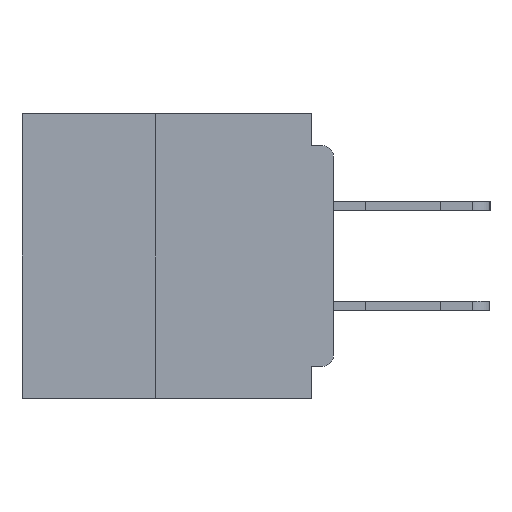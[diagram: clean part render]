
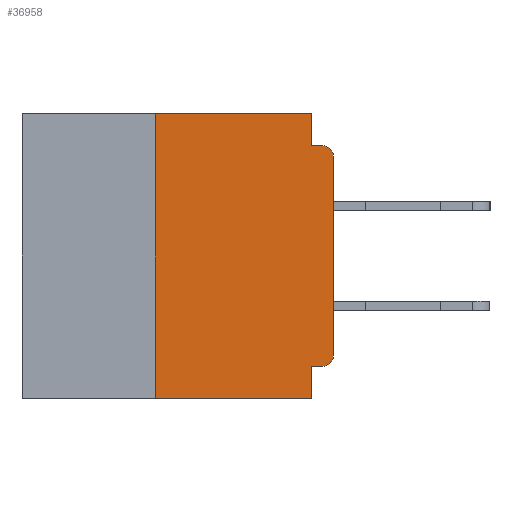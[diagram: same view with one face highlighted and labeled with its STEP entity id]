
A CAD part, left-side view. The second image highlights one B-rep face of the part: STEP entity #36958.
In plain terms, the highlighted planar face has unit normal (-1, 0, 0).
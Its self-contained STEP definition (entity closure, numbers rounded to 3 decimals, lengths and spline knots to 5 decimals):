
#415 = VECTOR ( 'NONE', #36513, 39.37008 ) ;
#615 = DIRECTION ( 'NONE',  ( 0., -1., 0. ) ) ;
#654 = CARTESIAN_POINT ( 'NONE',  ( 0., 0.015, -0.34 ) ) ;
#1583 = DIRECTION ( 'NONE',  ( -1., 0., 0. ) ) ;
#2540 = ORIENTED_EDGE ( 'NONE', *, *, #33725, .F. ) ;
#3178 = VECTOR ( 'NONE', #615, 39.37008 ) ;
#3676 = ORIENTED_EDGE ( 'NONE', *, *, #40113, .F. ) ;
#5214 = DIRECTION ( 'NONE',  ( 0., 0., 1. ) ) ;
#5276 = DIRECTION ( 'NONE',  ( 0., 0., -1. ) ) ;
#6387 = CARTESIAN_POINT ( 'NONE',  ( 0., 0.015, -0.355 ) ) ;
#6751 = CARTESIAN_POINT ( 'NONE',  ( 0., 0.031, 0. ) ) ;
#7031 = CARTESIAN_POINT ( 'NONE',  ( 0., 0.437, 0. ) ) ;
#7230 = DIRECTION ( 'NONE',  ( 0., 0., -1. ) ) ;
#7504 = LINE ( 'NONE', #15023, #29259 ) ;
#8085 = VERTEX_POINT ( 'NONE', #31874 ) ;
#8742 = ORIENTED_EDGE ( 'NONE', *, *, #43768, .T. ) ;
#8785 = EDGE_CURVE ( 'NONE', #26803, #26391, #31100, .T. ) ;
#8817 = CARTESIAN_POINT ( 'NONE',  ( 0., 0.25, 0. ) ) ;
#12615 = CARTESIAN_POINT ( 'NONE',  ( 0., 0.25, -0.4 ) ) ;
#13322 = LINE ( 'NONE', #33757, #37941 ) ;
#14015 = LINE ( 'NONE', #23815, #24891 ) ;
#15023 = CARTESIAN_POINT ( 'NONE',  ( 0., 0., -0.045 ) ) ;
#15478 = LINE ( 'NONE', #55989, #3178 ) ;
#17460 = LINE ( 'NONE', #35162, #52956 ) ;
#19173 = EDGE_CURVE ( 'NONE', #26803, #22892, #51169, .T. ) ;
#19683 = VERTEX_POINT ( 'NONE', #24675 ) ;
#20898 = CIRCLE ( 'NONE', #54994, 0.015 ) ;
#22050 = DIRECTION ( 'NONE',  ( 0., 0., -1. ) ) ;
#22139 = ORIENTED_EDGE ( 'NONE', *, *, #57718, .T. ) ;
#22577 = CARTESIAN_POINT ( 'NONE',  ( 0., 0.031, -0.355 ) ) ;
#22752 = CARTESIAN_POINT ( 'NONE',  ( 0., 0., 0. ) ) ;
#22892 = VERTEX_POINT ( 'NONE', #22577 ) ;
#23282 = VERTEX_POINT ( 'NONE', #6751 ) ;
#23600 = ORIENTED_EDGE ( 'NONE', *, *, #58479, .F. ) ;
#23815 = CARTESIAN_POINT ( 'NONE',  ( 0., 0.25, -0.4 ) ) ;
#24147 = ORIENTED_EDGE ( 'NONE', *, *, #53284, .F. ) ;
#24404 = EDGE_LOOP ( 'NONE', ( #22139, #8742, #3676, #28095, #24147, #23600, #30079, #2540, #34623, #55892 ) ) ;
#24675 = CARTESIAN_POINT ( 'NONE',  ( 0., 0.031, -0.045 ) ) ;
#24826 = CARTESIAN_POINT ( 'NONE',  ( 0., 0.031, -0.4 ) ) ;
#24891 = VECTOR ( 'NONE', #5214, 39.37008 ) ;
#25658 = PLANE ( 'NONE',  #49994 ) ;
#26391 = VERTEX_POINT ( 'NONE', #55522 ) ;
#26803 = VERTEX_POINT ( 'NONE', #6387 ) ;
#28095 = ORIENTED_EDGE ( 'NONE', *, *, #56971, .F. ) ;
#29259 = VECTOR ( 'NONE', #43020, 39.37008 ) ;
#29331 = CARTESIAN_POINT ( 'NONE',  ( 0., 0.015, -0.06 ) ) ;
#30079 = ORIENTED_EDGE ( 'NONE', *, *, #55406, .T. ) ;
#30431 = VERTEX_POINT ( 'NONE', #8817 ) ;
#30642 = CARTESIAN_POINT ( 'NONE',  ( 0., 0., -0.355 ) ) ;
#31100 = CIRCLE ( 'NONE', #58346, 0.015 ) ;
#31874 = CARTESIAN_POINT ( 'NONE',  ( 0., 0., -0.06 ) ) ;
#33011 = DIRECTION ( 'NONE',  ( -1., 0., 0. ) ) ;
#33725 = EDGE_CURVE ( 'NONE', #22892, #39547, #13322, .T. ) ;
#33757 = CARTESIAN_POINT ( 'NONE',  ( 0., 0.031, -0.4 ) ) ;
#33953 = DIRECTION ( 'NONE',  ( 0., 0., -1. ) ) ;
#34623 = ORIENTED_EDGE ( 'NONE', *, *, #19173, .F. ) ;
#34948 = DIRECTION ( 'NONE',  ( 1., 0., 0. ) ) ;
#35162 = CARTESIAN_POINT ( 'NONE',  ( 0., 0.437, -0.4 ) ) ;
#35773 = VERTEX_POINT ( 'NONE', #12615 ) ;
#36513 = DIRECTION ( 'NONE',  ( 0., 0., 1. ) ) ;
#36958 = ADVANCED_FACE ( 'NONE', ( #58576 ), #25658, .F. ) ;
#37941 = VECTOR ( 'NONE', #56765, 39.37008 ) ;
#39547 = VERTEX_POINT ( 'NONE', #24826 ) ;
#39834 = DIRECTION ( 'NONE',  ( 0., -1., 0. ) ) ;
#40113 = EDGE_CURVE ( 'NONE', #19683, #51002, #7504, .T. ) ;
#41059 = LINE ( 'NONE', #58980, #50426 ) ;
#43020 = DIRECTION ( 'NONE',  ( 0., -1., 0. ) ) ;
#43768 = EDGE_CURVE ( 'NONE', #8085, #51002, #20898, .T. ) ;
#44403 = DIRECTION ( 'NONE',  ( 0., 1., 0. ) ) ;
#45299 = LINE ( 'NONE', #22752, #415 ) ;
#49698 = VECTOR ( 'NONE', #44403, 39.37008 ) ;
#49994 = AXIS2_PLACEMENT_3D ( 'NONE', #7031, #34948, #7230 ) ;
#50426 = VECTOR ( 'NONE', #22050, 39.37008 ) ;
#51002 = VERTEX_POINT ( 'NONE', #59579 ) ;
#51169 = LINE ( 'NONE', #30642, #49698 ) ;
#52956 = VECTOR ( 'NONE', #39834, 39.37008 ) ;
#53284 = EDGE_CURVE ( 'NONE', #30431, #23282, #15478, .T. ) ;
#54994 = AXIS2_PLACEMENT_3D ( 'NONE', #29331, #1583, #33953 ) ;
#55406 = EDGE_CURVE ( 'NONE', #35773, #39547, #17460, .T. ) ;
#55522 = CARTESIAN_POINT ( 'NONE',  ( 0., 0., -0.34 ) ) ;
#55892 = ORIENTED_EDGE ( 'NONE', *, *, #8785, .T. ) ;
#55989 = CARTESIAN_POINT ( 'NONE',  ( 0., 0.437, 0. ) ) ;
#56765 = DIRECTION ( 'NONE',  ( 0., 0., -1. ) ) ;
#56971 = EDGE_CURVE ( 'NONE', #23282, #19683, #41059, .T. ) ;
#57718 = EDGE_CURVE ( 'NONE', #26391, #8085, #45299, .T. ) ;
#58346 = AXIS2_PLACEMENT_3D ( 'NONE', #654, #33011, #5276 ) ;
#58479 = EDGE_CURVE ( 'NONE', #35773, #30431, #14015, .T. ) ;
#58576 = FACE_OUTER_BOUND ( 'NONE', #24404, .T. ) ;
#58980 = CARTESIAN_POINT ( 'NONE',  ( 0., 0.031, 0. ) ) ;
#59579 = CARTESIAN_POINT ( 'NONE',  ( 0., 0.015, -0.045 ) ) ;
